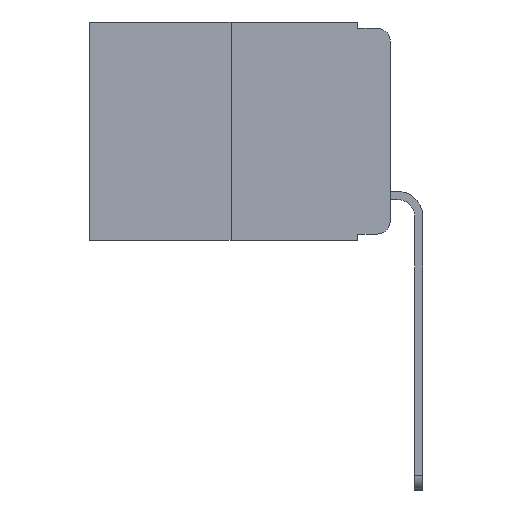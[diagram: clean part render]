
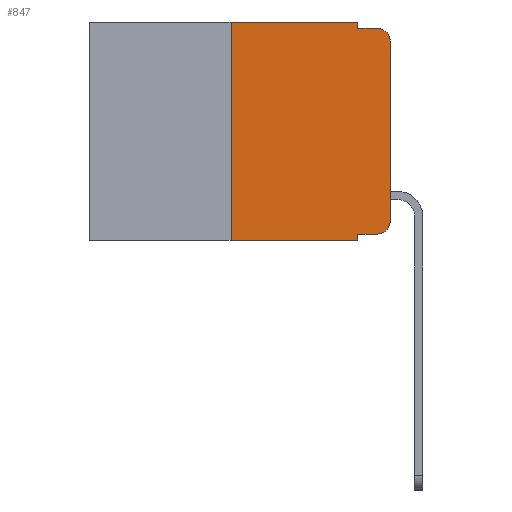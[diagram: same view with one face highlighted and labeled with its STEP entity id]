
A CAD part, left-side view. The second image highlights one B-rep face of the part: STEP entity #847.
In plain terms, the highlighted planar face has unit normal (-1, 0, 0).
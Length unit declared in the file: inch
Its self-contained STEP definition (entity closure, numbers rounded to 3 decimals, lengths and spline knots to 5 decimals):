
#847 = ADVANCED_FACE ( 'NONE', ( #14468 ), #16863, .F. ) ;
#853 = CARTESIAN_POINT ( 'NONE',  ( 0., 0.02, -0.333 ) ) ;
#907 = VECTOR ( 'NONE', #17097, 39.37008 ) ;
#1230 = LINE ( 'NONE', #12516, #16093 ) ;
#1241 = VERTEX_POINT ( 'NONE', #7219 ) ;
#1302 = CARTESIAN_POINT ( 'NONE',  ( 0., 0.051, -0.333 ) ) ;
#1363 = VERTEX_POINT ( 'NONE', #1999 ) ;
#1962 = EDGE_CURVE ( 'NONE', #17260, #14108, #6232, .T. ) ;
#1999 = CARTESIAN_POINT ( 'NONE',  ( 0., 0.051, -0.01 ) ) ;
#2083 = DIRECTION ( 'NONE',  ( 0., -1., 0. ) ) ;
#2131 = LINE ( 'NONE', #13488, #9527 ) ;
#2438 = CIRCLE ( 'NONE', #3152, 0.02 ) ;
#2711 = DIRECTION ( 'NONE',  ( 0., 0., -1. ) ) ;
#2934 = EDGE_CURVE ( 'NONE', #4007, #4856, #2438, .T. ) ;
#3094 = ORIENTED_EDGE ( 'NONE', *, *, #11871, .F. ) ;
#3102 = CARTESIAN_POINT ( 'NONE',  ( 0., 0.051, -0.333 ) ) ;
#3152 = AXIS2_PLACEMENT_3D ( 'NONE', #11954, #5802, #6367 ) ;
#3215 = VERTEX_POINT ( 'NONE', #12424 ) ;
#3295 = EDGE_CURVE ( 'NONE', #4856, #17260, #1230, .T. ) ;
#3421 = DIRECTION ( 'NONE',  ( 0., 0., -1. ) ) ;
#3538 = CARTESIAN_POINT ( 'NONE',  ( 0., 0.02, -0.01 ) ) ;
#3836 = ORIENTED_EDGE ( 'NONE', *, *, #17092, .F. ) ;
#4007 = VERTEX_POINT ( 'NONE', #853 ) ;
#4727 = LINE ( 'NONE', #8959, #16044 ) ;
#4742 = EDGE_CURVE ( 'NONE', #3215, #1241, #4727, .T. ) ;
#4772 = CARTESIAN_POINT ( 'NONE',  ( 0., 0.25, -0.343 ) ) ;
#4856 = VERTEX_POINT ( 'NONE', #5729 ) ;
#5069 = CARTESIAN_POINT ( 'NONE',  ( 0., 0.051, -0.01 ) ) ;
#5175 = DIRECTION ( 'NONE',  ( 0., -1., 0. ) ) ;
#5313 = VECTOR ( 'NONE', #2083, 39.37008 ) ;
#5597 = CARTESIAN_POINT ( 'NONE',  ( 0., 0.051, 0. ) ) ;
#5729 = CARTESIAN_POINT ( 'NONE',  ( 0., 0., -0.313 ) ) ;
#5802 = DIRECTION ( 'NONE',  ( -1., 0., 0. ) ) ;
#5947 = ORIENTED_EDGE ( 'NONE', *, *, #4742, .F. ) ;
#6144 = VECTOR ( 'NONE', #5175, 39.37008 ) ;
#6161 = ORIENTED_EDGE ( 'NONE', *, *, #8437, .F. ) ;
#6232 = CIRCLE ( 'NONE', #8591, 0.02 ) ;
#6367 = DIRECTION ( 'NONE',  ( 0., 0., -1. ) ) ;
#6981 = CARTESIAN_POINT ( 'NONE',  ( 0., 0.051, -0.343 ) ) ;
#7203 = LINE ( 'NONE', #13326, #14254 ) ;
#7219 = CARTESIAN_POINT ( 'NONE',  ( 0., 0.051, 0. ) ) ;
#7479 = ORIENTED_EDGE ( 'NONE', *, *, #2934, .T. ) ;
#7664 = ORIENTED_EDGE ( 'NONE', *, *, #3295, .T. ) ;
#7713 = DIRECTION ( 'NONE',  ( 0., 0., 1. ) ) ;
#7933 = CARTESIAN_POINT ( 'NONE',  ( 0., 0.473, 0. ) ) ;
#8091 = EDGE_CURVE ( 'NONE', #1241, #1363, #11066, .T. ) ;
#8437 = EDGE_CURVE ( 'NONE', #15009, #15633, #2131, .T. ) ;
#8591 = AXIS2_PLACEMENT_3D ( 'NONE', #14487, #15218, #2711 ) ;
#8959 = CARTESIAN_POINT ( 'NONE',  ( 0., 0.473, 0. ) ) ;
#9180 = LINE ( 'NONE', #5069, #5313 ) ;
#9460 = CARTESIAN_POINT ( 'NONE',  ( 0., 0., -0.03 ) ) ;
#9527 = VECTOR ( 'NONE', #3421, 39.37008 ) ;
#9696 = EDGE_CURVE ( 'NONE', #15009, #4007, #12549, .T. ) ;
#9970 = LINE ( 'NONE', #16414, #6144 ) ;
#11066 = LINE ( 'NONE', #5597, #17946 ) ;
#11871 = EDGE_CURVE ( 'NONE', #1363, #14108, #9180, .T. ) ;
#11873 = AXIS2_PLACEMENT_3D ( 'NONE', #7933, #16495, #16343 ) ;
#11954 = CARTESIAN_POINT ( 'NONE',  ( 0., 0.02, -0.313 ) ) ;
#12424 = CARTESIAN_POINT ( 'NONE',  ( 0., 0.25, 0. ) ) ;
#12495 = DIRECTION ( 'NONE',  ( 0., 0., 1. ) ) ;
#12516 = CARTESIAN_POINT ( 'NONE',  ( 0., 0., 0. ) ) ;
#12549 = LINE ( 'NONE', #1302, #907 ) ;
#13326 = CARTESIAN_POINT ( 'NONE',  ( 0., 0.25, 0. ) ) ;
#13345 = ORIENTED_EDGE ( 'NONE', *, *, #1962, .T. ) ;
#13488 = CARTESIAN_POINT ( 'NONE',  ( 0., 0.051, 0. ) ) ;
#14105 = DIRECTION ( 'NONE',  ( 0., 0., -1. ) ) ;
#14108 = VERTEX_POINT ( 'NONE', #3538 ) ;
#14157 = EDGE_CURVE ( 'NONE', #15943, #15633, #9970, .T. ) ;
#14254 = VECTOR ( 'NONE', #7713, 39.37008 ) ;
#14468 = FACE_OUTER_BOUND ( 'NONE', #16553, .T. ) ;
#14487 = CARTESIAN_POINT ( 'NONE',  ( 0., 0.02, -0.03 ) ) ;
#15009 = VERTEX_POINT ( 'NONE', #3102 ) ;
#15218 = DIRECTION ( 'NONE',  ( -1., 0., 0. ) ) ;
#15633 = VERTEX_POINT ( 'NONE', #6981 ) ;
#15875 = ORIENTED_EDGE ( 'NONE', *, *, #9696, .T. ) ;
#15943 = VERTEX_POINT ( 'NONE', #4772 ) ;
#16044 = VECTOR ( 'NONE', #17254, 39.37008 ) ;
#16093 = VECTOR ( 'NONE', #12495, 39.37008 ) ;
#16343 = DIRECTION ( 'NONE',  ( 0., 0., -1. ) ) ;
#16414 = CARTESIAN_POINT ( 'NONE',  ( 0., 0.473, -0.343 ) ) ;
#16495 = DIRECTION ( 'NONE',  ( 1., 0., 0. ) ) ;
#16553 = EDGE_LOOP ( 'NONE', ( #7664, #13345, #3094, #18221, #5947, #3836, #18214, #6161, #15875, #7479 ) ) ;
#16863 = PLANE ( 'NONE',  #11873 ) ;
#17092 = EDGE_CURVE ( 'NONE', #15943, #3215, #7203, .T. ) ;
#17097 = DIRECTION ( 'NONE',  ( 0., -1., 0. ) ) ;
#17254 = DIRECTION ( 'NONE',  ( 0., -1., 0. ) ) ;
#17260 = VERTEX_POINT ( 'NONE', #9460 ) ;
#17946 = VECTOR ( 'NONE', #14105, 39.37008 ) ;
#18214 = ORIENTED_EDGE ( 'NONE', *, *, #14157, .T. ) ;
#18221 = ORIENTED_EDGE ( 'NONE', *, *, #8091, .F. ) ;
